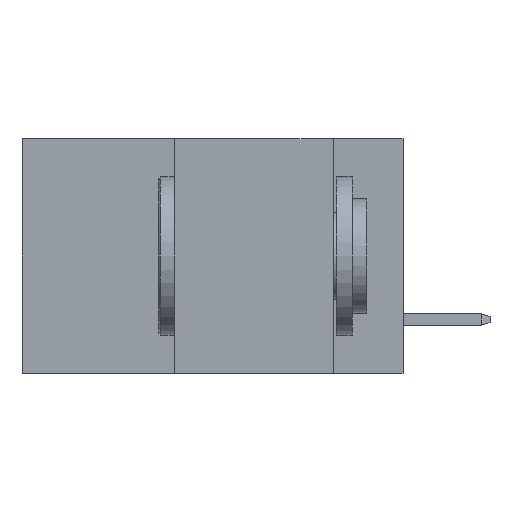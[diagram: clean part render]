
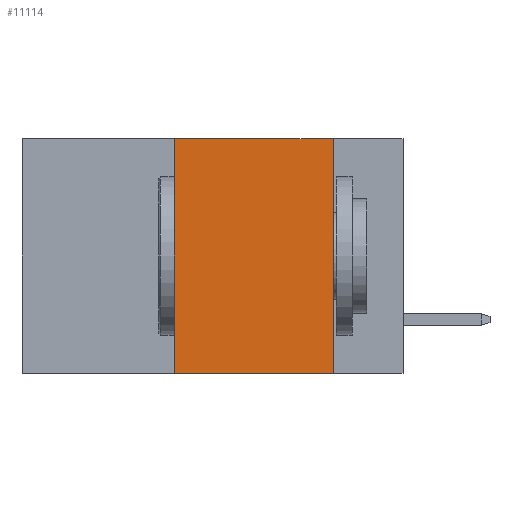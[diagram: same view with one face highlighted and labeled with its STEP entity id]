
A CAD part, left-side view. The second image highlights one B-rep face of the part: STEP entity #11114.
In plain terms, the highlighted planar face has unit normal (-1, 0, 0).
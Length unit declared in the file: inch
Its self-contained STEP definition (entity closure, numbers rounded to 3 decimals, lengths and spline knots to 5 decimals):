
#656 = VECTOR ( 'NONE', #14101, 39.37008 ) ;
#1470 = VECTOR ( 'NONE', #11421, 39.37008 ) ;
#1699 = EDGE_LOOP ( 'NONE', ( #8231, #5637, #9284, #7472 ) ) ;
#1950 = EDGE_CURVE ( 'NONE', #12684, #4462, #9274, .T. ) ;
#2262 = VERTEX_POINT ( 'NONE', #10135 ) ;
#2423 = DIRECTION ( 'NONE',  ( 0., -1., 0. ) ) ;
#3012 = FACE_OUTER_BOUND ( 'NONE', #1699, .T. ) ;
#3662 = CARTESIAN_POINT ( 'NONE',  ( 0., 0.36, 0. ) ) ;
#3737 = DIRECTION ( 'NONE',  ( 0., 0., 1. ) ) ;
#3753 = VERTEX_POINT ( 'NONE', #10878 ) ;
#4086 = CARTESIAN_POINT ( 'NONE',  ( 0., 0.6, -0.37 ) ) ;
#4306 = VECTOR ( 'NONE', #3737, 39.37008 ) ;
#4462 = VERTEX_POINT ( 'NONE', #11510 ) ;
#5281 = DIRECTION ( 'NONE',  ( 0., 0., -1. ) ) ;
#5531 = CARTESIAN_POINT ( 'NONE',  ( 0., 0.11, 0. ) ) ;
#5637 = ORIENTED_EDGE ( 'NONE', *, *, #1950, .F. ) ;
#6379 = CARTESIAN_POINT ( 'NONE',  ( 0., 0.6, 0. ) ) ;
#7182 = LINE ( 'NONE', #13826, #4306 ) ;
#7472 = ORIENTED_EDGE ( 'NONE', *, *, #8848, .T. ) ;
#8231 = ORIENTED_EDGE ( 'NONE', *, *, #10386, .F. ) ;
#8704 = LINE ( 'NONE', #4086, #656 ) ;
#8848 = EDGE_CURVE ( 'NONE', #2262, #3753, #8704, .T. ) ;
#9274 = LINE ( 'NONE', #12516, #11265 ) ;
#9284 = ORIENTED_EDGE ( 'NONE', *, *, #12726, .F. ) ;
#10135 = CARTESIAN_POINT ( 'NONE',  ( 0., 0.36, -0.37 ) ) ;
#10386 = EDGE_CURVE ( 'NONE', #4462, #3753, #13636, .T. ) ;
#10411 = AXIS2_PLACEMENT_3D ( 'NONE', #6379, #12958, #5281 ) ;
#10878 = CARTESIAN_POINT ( 'NONE',  ( 0., 0.11, -0.37 ) ) ;
#10957 = PLANE ( 'NONE',  #10411 ) ;
#11114 = ADVANCED_FACE ( 'NONE', ( #3012 ), #10957, .F. ) ;
#11265 = VECTOR ( 'NONE', #2423, 39.37008 ) ;
#11421 = DIRECTION ( 'NONE',  ( 0., 0., -1. ) ) ;
#11510 = CARTESIAN_POINT ( 'NONE',  ( 0., 0.11, 0. ) ) ;
#12516 = CARTESIAN_POINT ( 'NONE',  ( 0., 0.6, 0. ) ) ;
#12684 = VERTEX_POINT ( 'NONE', #3662 ) ;
#12726 = EDGE_CURVE ( 'NONE', #2262, #12684, #7182, .T. ) ;
#12958 = DIRECTION ( 'NONE',  ( 1., 0., 0. ) ) ;
#13636 = LINE ( 'NONE', #5531, #1470 ) ;
#13826 = CARTESIAN_POINT ( 'NONE',  ( 0., 0.36, 0. ) ) ;
#14101 = DIRECTION ( 'NONE',  ( 0., -1., 0. ) ) ;
